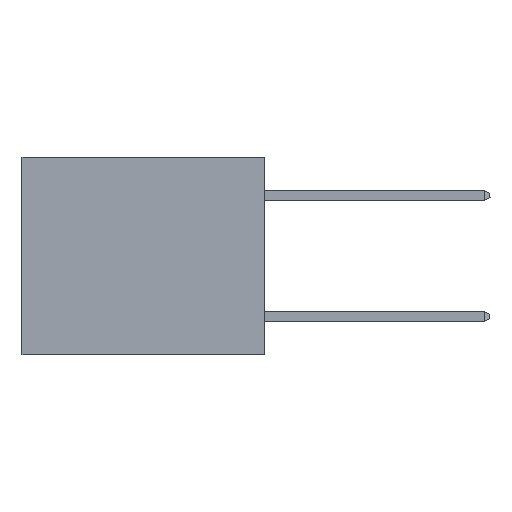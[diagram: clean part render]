
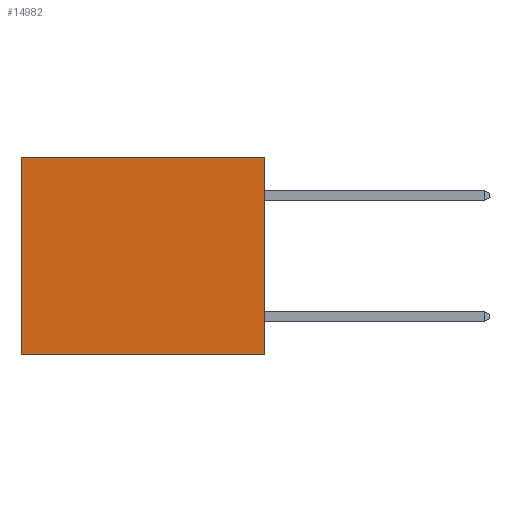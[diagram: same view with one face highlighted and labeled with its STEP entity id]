
A CAD part, left-side view. The second image highlights one B-rep face of the part: STEP entity #14982.
In plain terms, the highlighted planar face has unit normal (-1, 0, 0).
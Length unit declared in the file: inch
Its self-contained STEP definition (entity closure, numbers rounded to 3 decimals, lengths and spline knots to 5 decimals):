
#147 = CARTESIAN_POINT ( 'NONE',  ( 0.3165, 0.6, -0.49 ) ) ;
#1814 = DIRECTION ( 'NONE',  ( 1., 0., 0. ) ) ;
#3291 = CARTESIAN_POINT ( 'NONE',  ( 0.3165, 0., 0. ) ) ;
#5483 = VERTEX_POINT ( 'NONE', #3291 ) ;
#5693 = EDGE_CURVE ( 'NONE', #22164, #13517, #31523, .T. ) ;
#7118 = CARTESIAN_POINT ( 'NONE',  ( 0.3165, 0.6, 0. ) ) ;
#7288 = DIRECTION ( 'NONE',  ( 0., 0., -1. ) ) ;
#8789 = LINE ( 'NONE', #147, #26840 ) ;
#8961 = VECTOR ( 'NONE', #7288, 39.37008 ) ;
#9493 = EDGE_CURVE ( 'NONE', #5483, #22164, #28216, .T. ) ;
#10056 = AXIS2_PLACEMENT_3D ( 'NONE', #32137, #1814, #29737 ) ;
#10774 = CARTESIAN_POINT ( 'NONE',  ( 0.3165, 0., -0.49 ) ) ;
#12613 = CARTESIAN_POINT ( 'NONE',  ( 0.3165, 0., -0.49 ) ) ;
#13070 = LINE ( 'NONE', #32393, #29136 ) ;
#13517 = VERTEX_POINT ( 'NONE', #24157 ) ;
#14709 = CARTESIAN_POINT ( 'NONE',  ( 0.3165, 0., -0.49 ) ) ;
#14954 = DIRECTION ( 'NONE',  ( 0., 1., 0. ) ) ;
#14982 = ADVANCED_FACE ( 'NONE', ( #27265 ), #27246, .F. ) ;
#15922 = EDGE_LOOP ( 'NONE', ( #25273, #18790, #23999, #23061 ) ) ;
#18790 = ORIENTED_EDGE ( 'NONE', *, *, #5693, .F. ) ;
#22109 = EDGE_CURVE ( 'NONE', #24575, #13517, #8789, .T. ) ;
#22164 = VERTEX_POINT ( 'NONE', #12613 ) ;
#23061 = ORIENTED_EDGE ( 'NONE', *, *, #26028, .T. ) ;
#23268 = DIRECTION ( 'NONE',  ( 0., 1., 0. ) ) ;
#23999 = ORIENTED_EDGE ( 'NONE', *, *, #9493, .F. ) ;
#24157 = CARTESIAN_POINT ( 'NONE',  ( 0.3165, 0.6, -0.49 ) ) ;
#24575 = VERTEX_POINT ( 'NONE', #7118 ) ;
#24885 = VECTOR ( 'NONE', #23268, 39.37008 ) ;
#25273 = ORIENTED_EDGE ( 'NONE', *, *, #22109, .T. ) ;
#26028 = EDGE_CURVE ( 'NONE', #5483, #24575, #13070, .T. ) ;
#26840 = VECTOR ( 'NONE', #30273, 39.37008 ) ;
#27246 = PLANE ( 'NONE',  #10056 ) ;
#27265 = FACE_OUTER_BOUND ( 'NONE', #15922, .T. ) ;
#28216 = LINE ( 'NONE', #14709, #8961 ) ;
#29136 = VECTOR ( 'NONE', #14954, 39.37008 ) ;
#29737 = DIRECTION ( 'NONE',  ( 0., 0., -1. ) ) ;
#30273 = DIRECTION ( 'NONE',  ( 0., 0., -1. ) ) ;
#31523 = LINE ( 'NONE', #10774, #24885 ) ;
#32137 = CARTESIAN_POINT ( 'NONE',  ( 0.3165, 0., -0.49 ) ) ;
#32393 = CARTESIAN_POINT ( 'NONE',  ( 0.3165, 0., 0. ) ) ;
